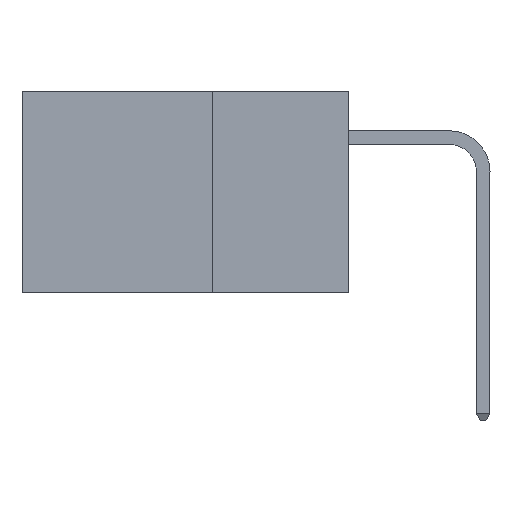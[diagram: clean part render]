
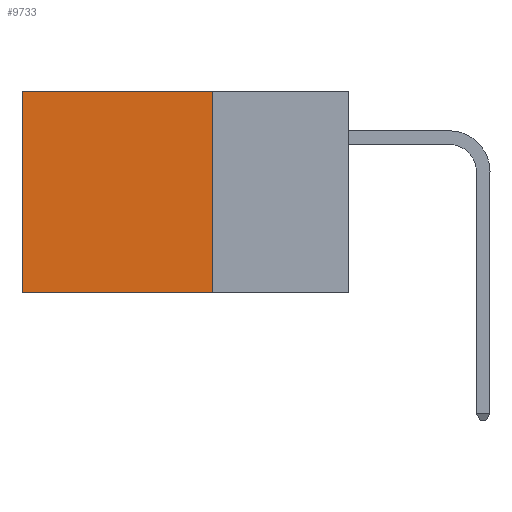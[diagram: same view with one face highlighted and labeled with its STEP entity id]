
A CAD part, left-side view. The second image highlights one B-rep face of the part: STEP entity #9733.
In plain terms, the highlighted planar face has unit normal (-1, 0, 0).
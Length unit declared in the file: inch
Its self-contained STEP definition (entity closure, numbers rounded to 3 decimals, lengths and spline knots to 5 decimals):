
#64 = ORIENTED_EDGE ( 'NONE', *, *, #2859, .T. ) ;
#1202 = ORIENTED_EDGE ( 'NONE', *, *, #14616, .F. ) ;
#1364 = VECTOR ( 'NONE', #21854, 39.37008 ) ;
#1614 = CARTESIAN_POINT ( 'NONE',  ( 0.2875, 0.6, 0. ) ) ;
#1761 = VECTOR ( 'NONE', #17752, 39.37008 ) ;
#1988 = EDGE_CURVE ( 'NONE', #24234, #9429, #11377, .T. ) ;
#2217 = FACE_OUTER_BOUND ( 'NONE', #17761, .T. ) ;
#2859 = EDGE_CURVE ( 'NONE', #20473, #9429, #22914, .T. ) ;
#3197 = VERTEX_POINT ( 'NONE', #11863 ) ;
#3813 = CARTESIAN_POINT ( 'NONE',  ( 0.2875, 0.25, 0. ) ) ;
#5085 = AXIS2_PLACEMENT_3D ( 'NONE', #19704, #7645, #21682 ) ;
#5300 = DIRECTION ( 'NONE',  ( 0., 0., -1. ) ) ;
#5882 = DIRECTION ( 'NONE',  ( 0., 1., 0. ) ) ;
#6818 = CARTESIAN_POINT ( 'NONE',  ( 0.2875, 0.25, -0.37 ) ) ;
#7645 = DIRECTION ( 'NONE',  ( 1., 0., 0. ) ) ;
#8243 = VECTOR ( 'NONE', #5300, 39.37008 ) ;
#9429 = VERTEX_POINT ( 'NONE', #12699 ) ;
#9733 = ADVANCED_FACE ( 'NONE', ( #2217 ), #23580, .F. ) ;
#11377 = LINE ( 'NONE', #18002, #1761 ) ;
#11863 = CARTESIAN_POINT ( 'NONE',  ( 0.2875, 0.25, 0. ) ) ;
#12699 = CARTESIAN_POINT ( 'NONE',  ( 0.2875, 0.6, -0.37 ) ) ;
#14616 = EDGE_CURVE ( 'NONE', #3197, #24234, #24192, .T. ) ;
#14692 = LINE ( 'NONE', #3813, #23426 ) ;
#17752 = DIRECTION ( 'NONE',  ( 0., 1., 0. ) ) ;
#17761 = EDGE_LOOP ( 'NONE', ( #64, #26045, #1202, #24268 ) ) ;
#18002 = CARTESIAN_POINT ( 'NONE',  ( 0.2875, 0.25, -0.37 ) ) ;
#18269 = EDGE_CURVE ( 'NONE', #3197, #20473, #14692, .T. ) ;
#19704 = CARTESIAN_POINT ( 'NONE',  ( 0.2875, 0.25, 0. ) ) ;
#20473 = VERTEX_POINT ( 'NONE', #1614 ) ;
#21448 = CARTESIAN_POINT ( 'NONE',  ( 0.2875, 0.25, 0. ) ) ;
#21682 = DIRECTION ( 'NONE',  ( 0., 0., -1. ) ) ;
#21854 = DIRECTION ( 'NONE',  ( 0., 0., -1. ) ) ;
#22088 = CARTESIAN_POINT ( 'NONE',  ( 0.2875, 0.6, 0. ) ) ;
#22914 = LINE ( 'NONE', #22088, #1364 ) ;
#23426 = VECTOR ( 'NONE', #5882, 39.37008 ) ;
#23580 = PLANE ( 'NONE',  #5085 ) ;
#24192 = LINE ( 'NONE', #21448, #8243 ) ;
#24234 = VERTEX_POINT ( 'NONE', #6818 ) ;
#24268 = ORIENTED_EDGE ( 'NONE', *, *, #18269, .T. ) ;
#26045 = ORIENTED_EDGE ( 'NONE', *, *, #1988, .F. ) ;
